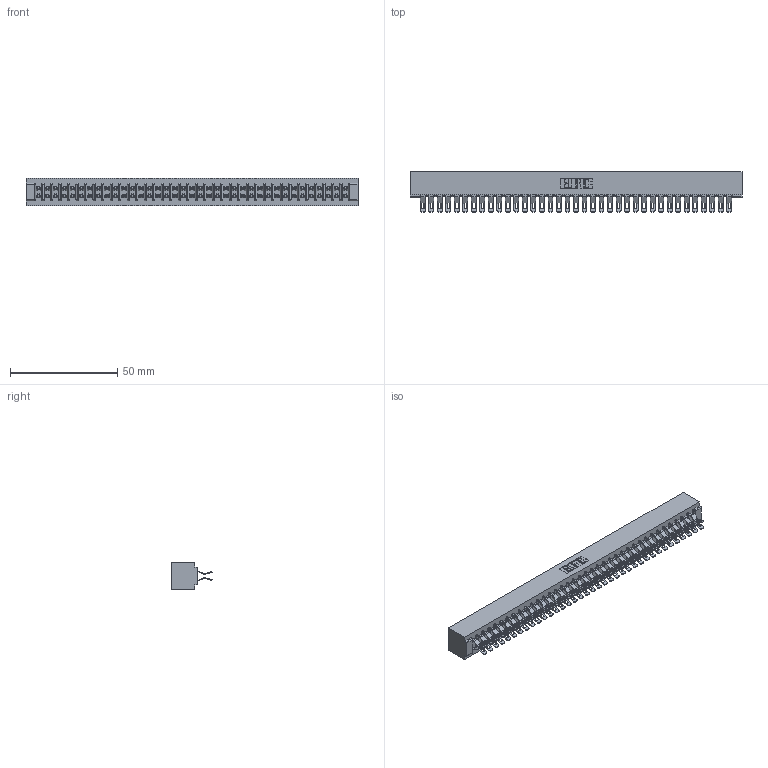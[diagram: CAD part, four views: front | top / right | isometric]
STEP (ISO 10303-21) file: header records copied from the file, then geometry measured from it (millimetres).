
FILE_DESCRIPTION (( 'STEP AP203' ), '1' );
FILE_NAME ('307-074-555-201.STEP', '2019-09-06T21:16:38', ( '' ), ( '' ), 'SwSTEP 2.0', 'SolidWorks 2016', '' );
FILE_SCHEMA (( 'CONFIG_CONTROL_DESIGN' ));
Length unit declared in the file: inch
Products named in the file (3): 307 Part_No Mounting Lugs; 307-290-001_555; 307-074-555-201
Assembly tree (75 placements, depth 2):
  307-074-555-201
    307 Part_No Mounting Lugs
    307-290-001_555  x74
Bounding box: 154.48 x 18.75 x 12.7 mm (x, y, z)
Volume: 17160 mm3; surface area: 22434 mm2
Topology: 75 solids, 75 shells, 4662 faces, 13693 edges, 8926 vertices
Faces by surface type: plane 2582, cylinder 2004, sphere 76
Entity records: 33779 total; most frequent: CARTESIAN_POINT 5529, ORIENTED_EDGE 5480, DIRECTION 5424, EDGE_CURVE 2740, LINE 2090, VECTOR 2090, VERTEX_POINT 1772, AXIS2_PLACEMENT_3D 1667
